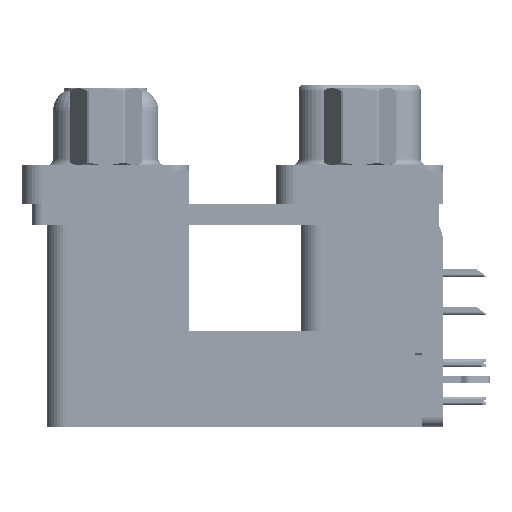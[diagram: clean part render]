
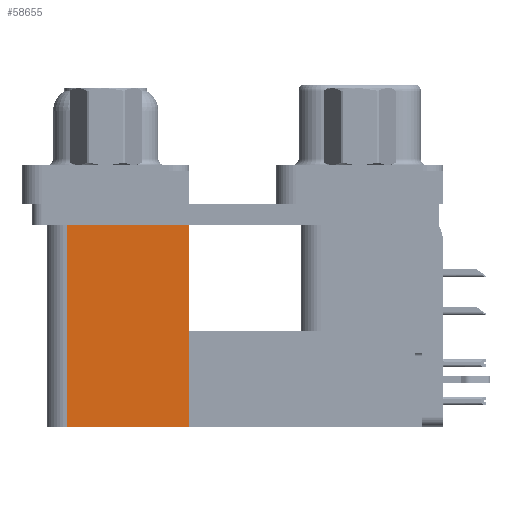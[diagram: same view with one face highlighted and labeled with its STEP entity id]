
A CAD part, left-side view. The second image highlights one B-rep face of the part: STEP entity #58655.
In plain terms, the highlighted planar face has unit normal (-1, 0, 0).
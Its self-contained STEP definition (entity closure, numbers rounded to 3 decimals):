
#435 = EDGE_CURVE ( 'NONE', #30385, #58108, #6754, .T. ) ;
#3202 = VECTOR ( 'NONE', #30438, 1000. ) ;
#3296 = DIRECTION ( 'NONE',  ( 0., 0., -1. ) ) ;
#5233 = LINE ( 'NONE', #38591, #16620 ) ;
#6324 = CARTESIAN_POINT ( 'NONE',  ( 3.7, 21.975, -19.2 ) ) ;
#6754 = LINE ( 'NONE', #25801, #10969 ) ;
#6757 = EDGE_CURVE ( 'NONE', #41577, #30385, #5233, .T. ) ;
#7353 = PLANE ( 'NONE',  #48954 ) ;
#10332 = VERTEX_POINT ( 'NONE', #16168 ) ;
#10969 = VECTOR ( 'NONE', #48865, 1000. ) ;
#13731 = CARTESIAN_POINT ( 'NONE',  ( 3.7, 21.975, -2.5 ) ) ;
#16168 = CARTESIAN_POINT ( 'NONE',  ( 3.7, 12.775, -2.5 ) ) ;
#16620 = VECTOR ( 'NONE', #49180, 1000. ) ;
#16729 = FACE_OUTER_BOUND ( 'NONE', #60688, .T. ) ;
#21735 = ORIENTED_EDGE ( 'NONE', *, *, #435, .F. ) ;
#23285 = ORIENTED_EDGE ( 'NONE', *, *, #27416, .T. ) ;
#25306 = CARTESIAN_POINT ( 'NONE',  ( 3.7, 12.775, -2.5 ) ) ;
#25762 = LINE ( 'NONE', #35724, #3202 ) ;
#25801 = CARTESIAN_POINT ( 'NONE',  ( 3.7, 21.975, -19.2 ) ) ;
#26442 = EDGE_CURVE ( 'NONE', #41577, #10332, #25762, .T. ) ;
#27416 = EDGE_CURVE ( 'NONE', #10332, #58108, #30602, .T. ) ;
#30385 = VERTEX_POINT ( 'NONE', #6324 ) ;
#30438 = DIRECTION ( 'NONE',  ( 0., 0., 1. ) ) ;
#30602 = LINE ( 'NONE', #25306, #38073 ) ;
#35724 = CARTESIAN_POINT ( 'NONE',  ( 3.7, 12.775, -19.2 ) ) ;
#35741 = DIRECTION ( 'NONE',  ( 1., 0., 0. ) ) ;
#38073 = VECTOR ( 'NONE', #44618, 1000. ) ;
#38403 = CARTESIAN_POINT ( 'NONE',  ( 3.7, 12.775, -19.2 ) ) ;
#38591 = CARTESIAN_POINT ( 'NONE',  ( 3.7, 12.775, -19.2 ) ) ;
#41577 = VERTEX_POINT ( 'NONE', #38403 ) ;
#44618 = DIRECTION ( 'NONE',  ( 0., 1., 0. ) ) ;
#48865 = DIRECTION ( 'NONE',  ( 0., 0., 1. ) ) ;
#48954 = AXIS2_PLACEMENT_3D ( 'NONE', #50696, #35741, #3296 ) ;
#49180 = DIRECTION ( 'NONE',  ( 0., 1., 0. ) ) ;
#50696 = CARTESIAN_POINT ( 'NONE',  ( 3.7, 12.775, -19.2 ) ) ;
#51710 = ORIENTED_EDGE ( 'NONE', *, *, #26442, .T. ) ;
#58108 = VERTEX_POINT ( 'NONE', #13731 ) ;
#58655 = ADVANCED_FACE ( 'NONE', ( #16729 ), #7353, .F. ) ;
#58819 = ORIENTED_EDGE ( 'NONE', *, *, #6757, .F. ) ;
#60688 = EDGE_LOOP ( 'NONE', ( #23285, #21735, #58819, #51710 ) ) ;
